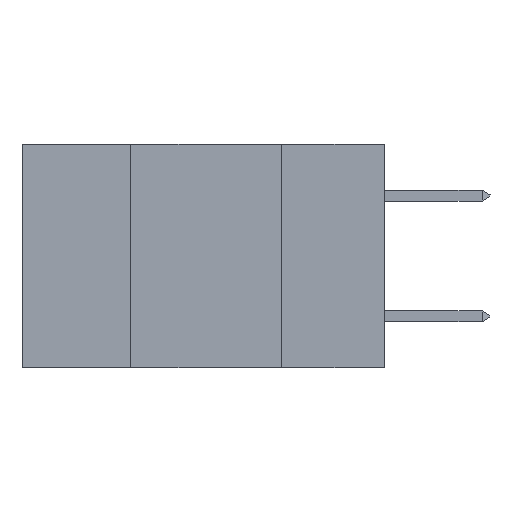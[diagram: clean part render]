
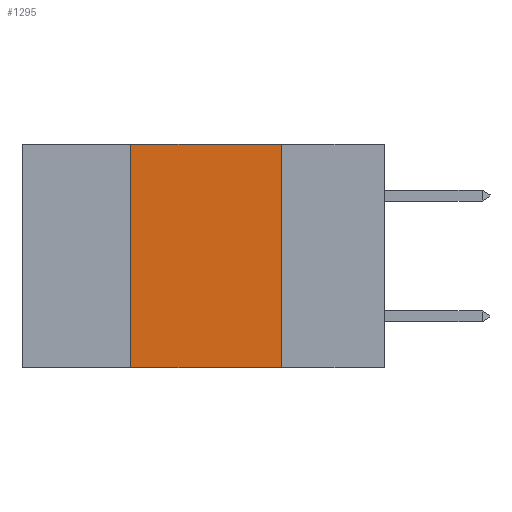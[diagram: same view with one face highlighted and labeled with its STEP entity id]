
A CAD part, left-side view. The second image highlights one B-rep face of the part: STEP entity #1295.
In plain terms, the highlighted planar face has unit normal (-1, 0, 0).
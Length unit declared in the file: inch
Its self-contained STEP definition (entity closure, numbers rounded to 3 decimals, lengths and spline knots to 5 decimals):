
#1295 = ADVANCED_FACE ( 'NONE', ( #26045 ), #27809, .F. ) ;
#1324 = DIRECTION ( 'NONE',  ( 0., 0., -1. ) ) ;
#1579 = DIRECTION ( 'NONE',  ( 0., -1., 0. ) ) ;
#2895 = VECTOR ( 'NONE', #15014, 39.37008 ) ;
#4045 = VECTOR ( 'NONE', #28556, 39.37008 ) ;
#4303 = EDGE_LOOP ( 'NONE', ( #7519, #17262, #15325, #9085 ) ) ;
#4805 = CARTESIAN_POINT ( 'NONE',  ( 0., 0.42, 0. ) ) ;
#4871 = EDGE_CURVE ( 'NONE', #18943, #20503, #15968, .T. ) ;
#5210 = AXIS2_PLACEMENT_3D ( 'NONE', #5530, #9832, #23166 ) ;
#5530 = CARTESIAN_POINT ( 'NONE',  ( 0., 0.6, 0. ) ) ;
#5772 = LINE ( 'NONE', #14481, #28549 ) ;
#5805 = CARTESIAN_POINT ( 'NONE',  ( 0., 0.42, 0. ) ) ;
#7519 = ORIENTED_EDGE ( 'NONE', *, *, #8683, .F. ) ;
#8492 = LINE ( 'NONE', #26351, #4045 ) ;
#8683 = EDGE_CURVE ( 'NONE', #20822, #16833, #5772, .T. ) ;
#9085 = ORIENTED_EDGE ( 'NONE', *, *, #28031, .T. ) ;
#9832 = DIRECTION ( 'NONE',  ( 1., 0., 0. ) ) ;
#9899 = CARTESIAN_POINT ( 'NONE',  ( 0., 0.42, -0.37 ) ) ;
#14481 = CARTESIAN_POINT ( 'NONE',  ( 0., 0.17, 0. ) ) ;
#14730 = CARTESIAN_POINT ( 'NONE',  ( 0., 0.6, -0.37 ) ) ;
#15014 = DIRECTION ( 'NONE',  ( 0., 0., 1. ) ) ;
#15252 = VECTOR ( 'NONE', #1579, 39.37008 ) ;
#15325 = ORIENTED_EDGE ( 'NONE', *, *, #4871, .F. ) ;
#15968 = LINE ( 'NONE', #5805, #2895 ) ;
#16833 = VERTEX_POINT ( 'NONE', #25078 ) ;
#17262 = ORIENTED_EDGE ( 'NONE', *, *, #25568, .F. ) ;
#18943 = VERTEX_POINT ( 'NONE', #9899 ) ;
#20503 = VERTEX_POINT ( 'NONE', #4805 ) ;
#20822 = VERTEX_POINT ( 'NONE', #21508 ) ;
#21508 = CARTESIAN_POINT ( 'NONE',  ( 0., 0.17, 0. ) ) ;
#23166 = DIRECTION ( 'NONE',  ( 0., 0., -1. ) ) ;
#25078 = CARTESIAN_POINT ( 'NONE',  ( 0., 0.17, -0.37 ) ) ;
#25568 = EDGE_CURVE ( 'NONE', #20503, #20822, #8492, .T. ) ;
#26045 = FACE_OUTER_BOUND ( 'NONE', #4303, .T. ) ;
#26351 = CARTESIAN_POINT ( 'NONE',  ( 0., 0.6, 0. ) ) ;
#27047 = LINE ( 'NONE', #14730, #15252 ) ;
#27809 = PLANE ( 'NONE',  #5210 ) ;
#28031 = EDGE_CURVE ( 'NONE', #18943, #16833, #27047, .T. ) ;
#28549 = VECTOR ( 'NONE', #1324, 39.37008 ) ;
#28556 = DIRECTION ( 'NONE',  ( 0., -1., 0. ) ) ;
